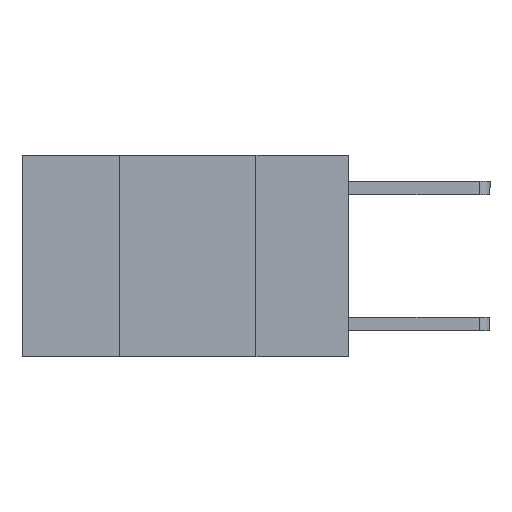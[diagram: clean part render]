
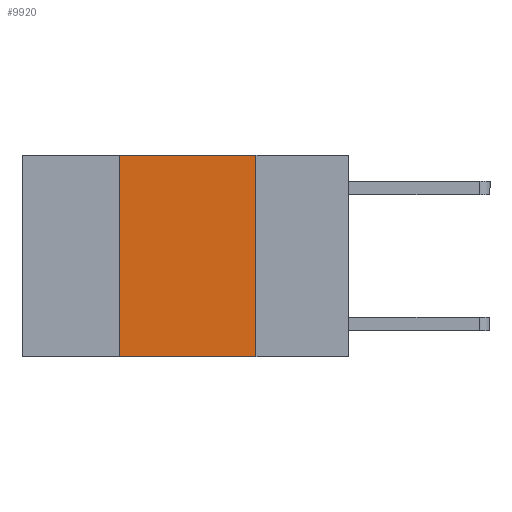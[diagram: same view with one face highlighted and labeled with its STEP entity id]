
A CAD part, left-side view. The second image highlights one B-rep face of the part: STEP entity #9920.
In plain terms, the highlighted planar face has unit normal (-1, 0, 0).
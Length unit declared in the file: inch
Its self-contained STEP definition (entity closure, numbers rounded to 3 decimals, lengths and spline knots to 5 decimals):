
#175 = VERTEX_POINT ( 'NONE', #1940 ) ;
#241 = VERTEX_POINT ( 'NONE', #1890 ) ;
#518 = DIRECTION ( 'NONE',  ( 0., 0., -1. ) ) ;
#870 = VERTEX_POINT ( 'NONE', #7359 ) ;
#1246 = ORIENTED_EDGE ( 'NONE', *, *, #7923, .T. ) ;
#1462 = CARTESIAN_POINT ( 'NONE',  ( 0., 0.17, 0. ) ) ;
#1874 = AXIS2_PLACEMENT_3D ( 'NONE', #3713, #6815, #2957 ) ;
#1890 = CARTESIAN_POINT ( 'NONE',  ( 0., 0.17, -0.37 ) ) ;
#1940 = CARTESIAN_POINT ( 'NONE',  ( 0., 0.42, -0.37 ) ) ;
#2400 = VECTOR ( 'NONE', #4312, 39.37008 ) ;
#2596 = VECTOR ( 'NONE', #3563, 39.37008 ) ;
#2802 = CARTESIAN_POINT ( 'NONE',  ( 0., 0.42, 0. ) ) ;
#2957 = DIRECTION ( 'NONE',  ( 0., 0., -1. ) ) ;
#3114 = EDGE_LOOP ( 'NONE', ( #9892, #9465, #6188, #1246 ) ) ;
#3563 = DIRECTION ( 'NONE',  ( 0., 0., 1. ) ) ;
#3568 = EDGE_CURVE ( 'NONE', #175, #870, #8145, .T. ) ;
#3713 = CARTESIAN_POINT ( 'NONE',  ( 0., 0.6, 0. ) ) ;
#3771 = LINE ( 'NONE', #1462, #4647 ) ;
#4312 = DIRECTION ( 'NONE',  ( 0., -1., 0. ) ) ;
#4515 = PLANE ( 'NONE',  #1874 ) ;
#4647 = VECTOR ( 'NONE', #518, 39.37008 ) ;
#5125 = CARTESIAN_POINT ( 'NONE',  ( 0., 0.6, -0.37 ) ) ;
#5724 = LINE ( 'NONE', #5125, #2400 ) ;
#5965 = EDGE_CURVE ( 'NONE', #870, #6035, #8556, .T. ) ;
#6035 = VERTEX_POINT ( 'NONE', #9563 ) ;
#6188 = ORIENTED_EDGE ( 'NONE', *, *, #3568, .F. ) ;
#6815 = DIRECTION ( 'NONE',  ( 1., 0., 0. ) ) ;
#7313 = EDGE_CURVE ( 'NONE', #6035, #241, #3771, .T. ) ;
#7359 = CARTESIAN_POINT ( 'NONE',  ( 0., 0.42, 0. ) ) ;
#7401 = DIRECTION ( 'NONE',  ( 0., -1., 0. ) ) ;
#7584 = FACE_OUTER_BOUND ( 'NONE', #3114, .T. ) ;
#7923 = EDGE_CURVE ( 'NONE', #175, #241, #5724, .T. ) ;
#8145 = LINE ( 'NONE', #2802, #2596 ) ;
#8556 = LINE ( 'NONE', #9116, #9996 ) ;
#9116 = CARTESIAN_POINT ( 'NONE',  ( 0., 0.6, 0. ) ) ;
#9465 = ORIENTED_EDGE ( 'NONE', *, *, #5965, .F. ) ;
#9563 = CARTESIAN_POINT ( 'NONE',  ( 0., 0.17, 0. ) ) ;
#9892 = ORIENTED_EDGE ( 'NONE', *, *, #7313, .F. ) ;
#9920 = ADVANCED_FACE ( 'NONE', ( #7584 ), #4515, .F. ) ;
#9996 = VECTOR ( 'NONE', #7401, 39.37008 ) ;
